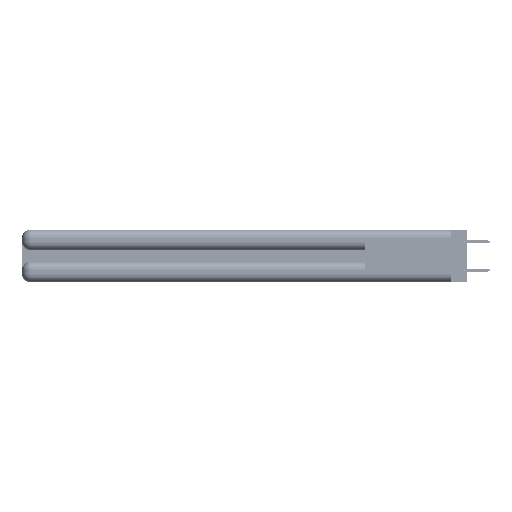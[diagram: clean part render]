
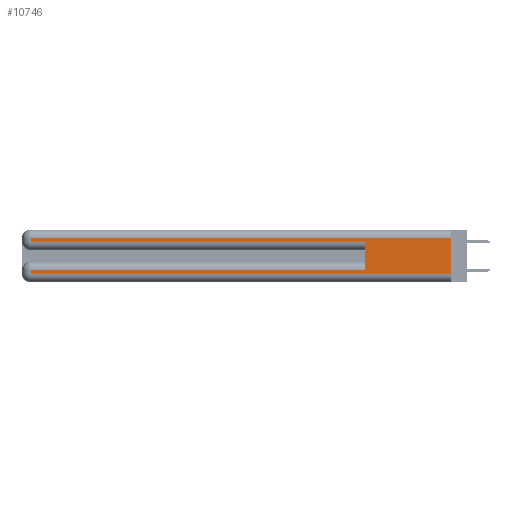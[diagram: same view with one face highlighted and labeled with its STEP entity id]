
A CAD part, left-side view. The second image highlights one B-rep face of the part: STEP entity #10746.
In plain terms, the highlighted planar face has unit normal (-1, 0, 0).
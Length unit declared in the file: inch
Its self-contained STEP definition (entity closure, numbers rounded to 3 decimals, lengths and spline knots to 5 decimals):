
#612 = CARTESIAN_POINT ( 'NONE',  ( 0., 2.94, 0.37 ) ) ;
#2082 = CARTESIAN_POINT ( 'NONE',  ( 0., 2.94, 0.06 ) ) ;
#2134 = CARTESIAN_POINT ( 'NONE',  ( 0., 0., 0.37 ) ) ;
#2805 = VECTOR ( 'NONE', #8372, 39.37008 ) ;
#4011 = CARTESIAN_POINT ( 'NONE',  ( 0., 0., 0.06 ) ) ;
#4031 = AXIS2_PLACEMENT_3D ( 'NONE', #27566, #7241, #23117 ) ;
#5022 = CARTESIAN_POINT ( 'NONE',  ( 0., 0.6, 0.085 ) ) ;
#5515 = FACE_OUTER_BOUND ( 'NONE', #48146, .T. ) ;
#5808 = ORIENTED_EDGE ( 'NONE', *, *, #12164, .T. ) ;
#6207 = VERTEX_POINT ( 'NONE', #38674 ) ;
#6632 = CARTESIAN_POINT ( 'NONE',  ( 0., 0., 0.285 ) ) ;
#7241 = DIRECTION ( 'NONE',  ( 1., 0., 0. ) ) ;
#7253 = VECTOR ( 'NONE', #33105, 39.37008 ) ;
#7930 = CARTESIAN_POINT ( 'NONE',  ( 0., 0., 0.06 ) ) ;
#8372 = DIRECTION ( 'NONE',  ( 0., 1., 0. ) ) ;
#9140 = LINE ( 'NONE', #4011, #7253 ) ;
#10172 = EDGE_CURVE ( 'NONE', #32160, #6207, #37500, .T. ) ;
#10683 = VERTEX_POINT ( 'NONE', #43779 ) ;
#10746 = ADVANCED_FACE ( 'NONE', ( #5515 ), #30953, .F. ) ;
#11081 = LINE ( 'NONE', #32291, #2805 ) ;
#11385 = DIRECTION ( 'NONE',  ( 0., 0., 1. ) ) ;
#11559 = CARTESIAN_POINT ( 'NONE',  ( 0., 0.6, 0.145 ) ) ;
#11607 = EDGE_CURVE ( 'NONE', #23083, #10683, #36706, .T. ) ;
#12164 = EDGE_CURVE ( 'NONE', #26387, #23083, #11081, .T. ) ;
#13172 = ORIENTED_EDGE ( 'NONE', *, *, #52594, .T. ) ;
#14079 = DIRECTION ( 'NONE',  ( 0., 0., -1. ) ) ;
#15809 = ORIENTED_EDGE ( 'NONE', *, *, #34135, .T. ) ;
#15850 = ORIENTED_EDGE ( 'NONE', *, *, #37527, .F. ) ;
#16089 = LINE ( 'NONE', #50750, #42852 ) ;
#16944 = VECTOR ( 'NONE', #45134, 39.37008 ) ;
#17694 = ORIENTED_EDGE ( 'NONE', *, *, #11607, .T. ) ;
#19481 = CARTESIAN_POINT ( 'NONE',  ( 0., 2.94, 0.31 ) ) ;
#23083 = VERTEX_POINT ( 'NONE', #19481 ) ;
#23117 = DIRECTION ( 'NONE',  ( 0., 0., -1. ) ) ;
#24921 = LINE ( 'NONE', #47547, #42183 ) ;
#25029 = ORIENTED_EDGE ( 'NONE', *, *, #10172, .F. ) ;
#26228 = CARTESIAN_POINT ( 'NONE',  ( 0., 2.94, 0.085 ) ) ;
#26387 = VERTEX_POINT ( 'NONE', #28702 ) ;
#26571 = DIRECTION ( 'NONE',  ( 0., 1., 0. ) ) ;
#26911 = DIRECTION ( 'NONE',  ( 0., 0., -1. ) ) ;
#27493 = DIRECTION ( 'NONE',  ( 0., -1., 0. ) ) ;
#27566 = CARTESIAN_POINT ( 'NONE',  ( 0., 0., 0.37 ) ) ;
#27942 = VECTOR ( 'NONE', #11385, 39.37008 ) ;
#28702 = CARTESIAN_POINT ( 'NONE',  ( 0., 0., 0.31 ) ) ;
#30953 = PLANE ( 'NONE',  #4031 ) ;
#31058 = VECTOR ( 'NONE', #26911, 39.37008 ) ;
#32160 = VERTEX_POINT ( 'NONE', #5022 ) ;
#32291 = CARTESIAN_POINT ( 'NONE',  ( 0., 0., 0.31 ) ) ;
#33105 = DIRECTION ( 'NONE',  ( 0., -1., 0. ) ) ;
#33775 = VERTEX_POINT ( 'NONE', #7930 ) ;
#34135 = EDGE_CURVE ( 'NONE', #41926, #52191, #16089, .T. ) ;
#36706 = LINE ( 'NONE', #612, #16944 ) ;
#37500 = LINE ( 'NONE', #11559, #27942 ) ;
#37527 = EDGE_CURVE ( 'NONE', #26387, #33775, #41935, .T. ) ;
#38674 = CARTESIAN_POINT ( 'NONE',  ( 0., 0.6, 0.285 ) ) ;
#41585 = ORIENTED_EDGE ( 'NONE', *, *, #42069, .T. ) ;
#41926 = VERTEX_POINT ( 'NONE', #26228 ) ;
#41935 = LINE ( 'NONE', #2134, #31058 ) ;
#42069 = EDGE_CURVE ( 'NONE', #32160, #41926, #24921, .T. ) ;
#42183 = VECTOR ( 'NONE', #26571, 39.37008 ) ;
#42852 = VECTOR ( 'NONE', #14079, 39.37008 ) ;
#43779 = CARTESIAN_POINT ( 'NONE',  ( 0., 2.94, 0.285 ) ) ;
#44340 = LINE ( 'NONE', #6632, #50012 ) ;
#45134 = DIRECTION ( 'NONE',  ( 0., 0., -1. ) ) ;
#45389 = EDGE_CURVE ( 'NONE', #10683, #6207, #44340, .T. ) ;
#47547 = CARTESIAN_POINT ( 'NONE',  ( 0., 0., 0.085 ) ) ;
#48146 = EDGE_LOOP ( 'NONE', ( #15850, #5808, #17694, #48354, #25029, #41585, #15809, #13172 ) ) ;
#48354 = ORIENTED_EDGE ( 'NONE', *, *, #45389, .T. ) ;
#50012 = VECTOR ( 'NONE', #27493, 39.37008 ) ;
#50750 = CARTESIAN_POINT ( 'NONE',  ( 0., 2.94, 0.37 ) ) ;
#52191 = VERTEX_POINT ( 'NONE', #2082 ) ;
#52594 = EDGE_CURVE ( 'NONE', #52191, #33775, #9140, .T. ) ;
